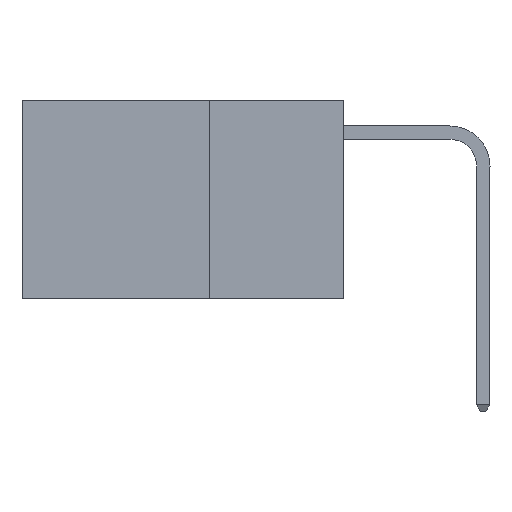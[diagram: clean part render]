
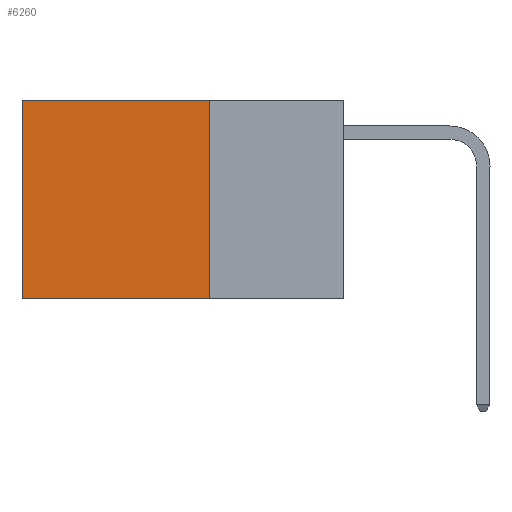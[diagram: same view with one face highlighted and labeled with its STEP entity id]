
A CAD part, left-side view. The second image highlights one B-rep face of the part: STEP entity #6260.
In plain terms, the highlighted planar face has unit normal (-1, 0, 0).
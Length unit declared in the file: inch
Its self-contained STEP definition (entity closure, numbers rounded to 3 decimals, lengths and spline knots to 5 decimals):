
#207 = DIRECTION ( 'NONE',  ( 0., 0., -1. ) ) ;
#425 = CARTESIAN_POINT ( 'NONE',  ( 0.2625, 0.6, -0.37 ) ) ;
#2127 = EDGE_CURVE ( 'NONE', #14909, #19137, #15169, .T. ) ;
#2540 = CARTESIAN_POINT ( 'NONE',  ( 0.2625, 0.25, 0. ) ) ;
#3129 = LINE ( 'NONE', #15883, #12685 ) ;
#4149 = CARTESIAN_POINT ( 'NONE',  ( 0.2625, 0.25, -0.37 ) ) ;
#4554 = VERTEX_POINT ( 'NONE', #2540 ) ;
#4922 = DIRECTION ( 'NONE',  ( 0., 1., 0. ) ) ;
#4976 = ORIENTED_EDGE ( 'NONE', *, *, #15609, .F. ) ;
#5129 = LINE ( 'NONE', #24530, #19181 ) ;
#5468 = VECTOR ( 'NONE', #18978, 39.37008 ) ;
#5546 = DIRECTION ( 'NONE',  ( 0., 0., -1. ) ) ;
#5611 = AXIS2_PLACEMENT_3D ( 'NONE', #23052, #11613, #207 ) ;
#6260 = ADVANCED_FACE ( 'NONE', ( #12846 ), #9687, .F. ) ;
#7535 = CARTESIAN_POINT ( 'NONE',  ( 0.2625, 0.25, 0. ) ) ;
#9687 = PLANE ( 'NONE',  #5611 ) ;
#9880 = EDGE_LOOP ( 'NONE', ( #17071, #12022, #4976, #16181 ) ) ;
#10085 = VECTOR ( 'NONE', #4922, 39.37008 ) ;
#10706 = EDGE_CURVE ( 'NONE', #4554, #11420, #21282, .T. ) ;
#11420 = VERTEX_POINT ( 'NONE', #17235 ) ;
#11613 = DIRECTION ( 'NONE',  ( 1., 0., 0. ) ) ;
#12022 = ORIENTED_EDGE ( 'NONE', *, *, #2127, .F. ) ;
#12685 = VECTOR ( 'NONE', #17850, 39.37008 ) ;
#12846 = FACE_OUTER_BOUND ( 'NONE', #9880, .T. ) ;
#14909 = VERTEX_POINT ( 'NONE', #4149 ) ;
#15169 = LINE ( 'NONE', #18958, #10085 ) ;
#15609 = EDGE_CURVE ( 'NONE', #4554, #14909, #3129, .T. ) ;
#15883 = CARTESIAN_POINT ( 'NONE',  ( 0.2625, 0.25, 0. ) ) ;
#16181 = ORIENTED_EDGE ( 'NONE', *, *, #10706, .T. ) ;
#17071 = ORIENTED_EDGE ( 'NONE', *, *, #20794, .T. ) ;
#17235 = CARTESIAN_POINT ( 'NONE',  ( 0.2625, 0.6, 0. ) ) ;
#17850 = DIRECTION ( 'NONE',  ( 0., 0., -1. ) ) ;
#18958 = CARTESIAN_POINT ( 'NONE',  ( 0.2625, 0.25, -0.37 ) ) ;
#18978 = DIRECTION ( 'NONE',  ( 0., 1., 0. ) ) ;
#19137 = VERTEX_POINT ( 'NONE', #425 ) ;
#19181 = VECTOR ( 'NONE', #5546, 39.37008 ) ;
#20794 = EDGE_CURVE ( 'NONE', #11420, #19137, #5129, .T. ) ;
#21282 = LINE ( 'NONE', #7535, #5468 ) ;
#23052 = CARTESIAN_POINT ( 'NONE',  ( 0.2625, 0.25, 0. ) ) ;
#24530 = CARTESIAN_POINT ( 'NONE',  ( 0.2625, 0.6, 0. ) ) ;
